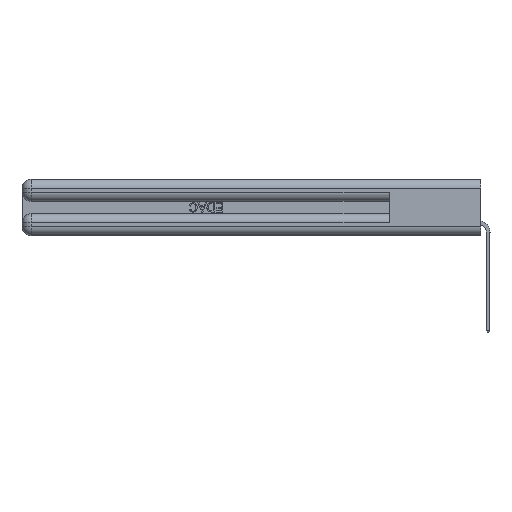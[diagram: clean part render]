
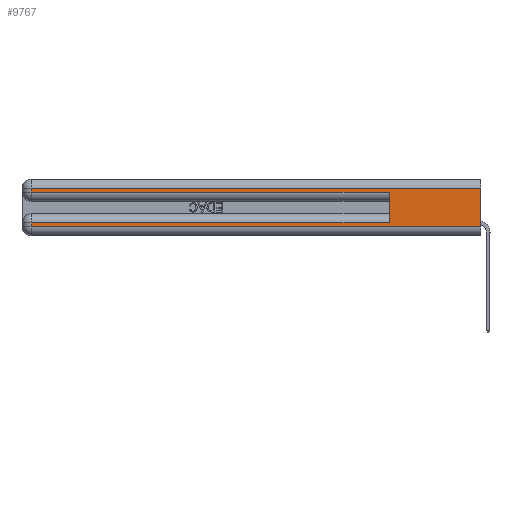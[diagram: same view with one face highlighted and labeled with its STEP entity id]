
A CAD part, left-side view. The second image highlights one B-rep face of the part: STEP entity #9767.
In plain terms, the highlighted planar face has unit normal (-1, 0, 0).
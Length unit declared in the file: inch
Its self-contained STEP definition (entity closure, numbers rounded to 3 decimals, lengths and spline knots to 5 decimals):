
#110 = DIRECTION ( 'NONE',  ( 0., 0., -1. ) ) ;
#471 = ORIENTED_EDGE ( 'NONE', *, *, #6741, .T. ) ;
#808 = DIRECTION ( 'NONE',  ( 0., 1., 0. ) ) ;
#860 = EDGE_LOOP ( 'NONE', ( #19136, #29811, #8137, #3269, #7323, #25403, #471, #20697 ) ) ;
#1047 = CARTESIAN_POINT ( 'NONE',  ( 0., 2.94, 0.285 ) ) ;
#1325 = DIRECTION ( 'NONE',  ( 0., 0., -1. ) ) ;
#2353 = LINE ( 'NONE', #32617, #8210 ) ;
#2904 = CARTESIAN_POINT ( 'NONE',  ( 0., 0., 0.31 ) ) ;
#3269 = ORIENTED_EDGE ( 'NONE', *, *, #11920, .T. ) ;
#3453 = LINE ( 'NONE', #23796, #22189 ) ;
#4743 = CARTESIAN_POINT ( 'NONE',  ( 0., 0., 0.06 ) ) ;
#4805 = VERTEX_POINT ( 'NONE', #20399 ) ;
#5002 = LINE ( 'NONE', #15740, #18308 ) ;
#5163 = DIRECTION ( 'NONE',  ( 0., 1., 0. ) ) ;
#5506 = EDGE_CURVE ( 'NONE', #16180, #24218, #18755, .T. ) ;
#5620 = CARTESIAN_POINT ( 'NONE',  ( 0., 2.94, 0.06 ) ) ;
#6741 = EDGE_CURVE ( 'NONE', #19125, #13672, #11474, .T. ) ;
#7008 = VERTEX_POINT ( 'NONE', #27157 ) ;
#7323 = ORIENTED_EDGE ( 'NONE', *, *, #32659, .F. ) ;
#7396 = VECTOR ( 'NONE', #33219, 39.37008 ) ;
#8137 = ORIENTED_EDGE ( 'NONE', *, *, #32264, .T. ) ;
#8210 = VECTOR ( 'NONE', #23501, 39.37008 ) ;
#8290 = VECTOR ( 'NONE', #28576, 39.37008 ) ;
#9767 = ADVANCED_FACE ( 'NONE', ( #28281 ), #32819, .F. ) ;
#10044 = LINE ( 'NONE', #4743, #26660 ) ;
#10461 = VERTEX_POINT ( 'NONE', #1047 ) ;
#10811 = LINE ( 'NONE', #17543, #8290 ) ;
#11448 = DIRECTION ( 'NONE',  ( 1., 0., 0. ) ) ;
#11470 = EDGE_CURVE ( 'NONE', #16180, #14754, #22353, .T. ) ;
#11474 = LINE ( 'NONE', #33855, #34330 ) ;
#11920 = EDGE_CURVE ( 'NONE', #10461, #4805, #2353, .T. ) ;
#13672 = VERTEX_POINT ( 'NONE', #5620 ) ;
#14106 = CARTESIAN_POINT ( 'NONE',  ( 0., 0., 0.37 ) ) ;
#14754 = VERTEX_POINT ( 'NONE', #23973 ) ;
#14987 = CARTESIAN_POINT ( 'NONE',  ( 0., 0., 0.37 ) ) ;
#15740 = CARTESIAN_POINT ( 'NONE',  ( 0., 2.94, 0.37 ) ) ;
#16180 = VERTEX_POINT ( 'NONE', #29236 ) ;
#17543 = CARTESIAN_POINT ( 'NONE',  ( 0., 0.6, 0.145 ) ) ;
#18182 = AXIS2_PLACEMENT_3D ( 'NONE', #14106, #11448, #1325 ) ;
#18308 = VECTOR ( 'NONE', #110, 39.37008 ) ;
#18755 = LINE ( 'NONE', #2904, #32092 ) ;
#19125 = VERTEX_POINT ( 'NONE', #25546 ) ;
#19136 = ORIENTED_EDGE ( 'NONE', *, *, #11470, .F. ) ;
#19444 = EDGE_CURVE ( 'NONE', #7008, #19125, #3453, .T. ) ;
#20399 = CARTESIAN_POINT ( 'NONE',  ( 0., 0.6, 0.285 ) ) ;
#20570 = DIRECTION ( 'NONE',  ( 0., -1., 0. ) ) ;
#20646 = DIRECTION ( 'NONE',  ( 0., 0., -1. ) ) ;
#20697 = ORIENTED_EDGE ( 'NONE', *, *, #27111, .T. ) ;
#22189 = VECTOR ( 'NONE', #5163, 39.37008 ) ;
#22353 = LINE ( 'NONE', #14987, #7396 ) ;
#22760 = CARTESIAN_POINT ( 'NONE',  ( 0., 2.94, 0.31 ) ) ;
#23501 = DIRECTION ( 'NONE',  ( 0., -1., 0. ) ) ;
#23796 = CARTESIAN_POINT ( 'NONE',  ( 0., 0., 0.085 ) ) ;
#23973 = CARTESIAN_POINT ( 'NONE',  ( 0., 0., 0.06 ) ) ;
#24218 = VERTEX_POINT ( 'NONE', #22760 ) ;
#25403 = ORIENTED_EDGE ( 'NONE', *, *, #19444, .T. ) ;
#25546 = CARTESIAN_POINT ( 'NONE',  ( 0., 2.94, 0.085 ) ) ;
#26660 = VECTOR ( 'NONE', #20570, 39.37008 ) ;
#27111 = EDGE_CURVE ( 'NONE', #13672, #14754, #10044, .T. ) ;
#27157 = CARTESIAN_POINT ( 'NONE',  ( 0., 0.6, 0.085 ) ) ;
#28281 = FACE_OUTER_BOUND ( 'NONE', #860, .T. ) ;
#28576 = DIRECTION ( 'NONE',  ( 0., 0., 1. ) ) ;
#29236 = CARTESIAN_POINT ( 'NONE',  ( 0., 0., 0.31 ) ) ;
#29811 = ORIENTED_EDGE ( 'NONE', *, *, #5506, .T. ) ;
#32092 = VECTOR ( 'NONE', #808, 39.37008 ) ;
#32264 = EDGE_CURVE ( 'NONE', #24218, #10461, #5002, .T. ) ;
#32617 = CARTESIAN_POINT ( 'NONE',  ( 0., 0., 0.285 ) ) ;
#32659 = EDGE_CURVE ( 'NONE', #7008, #4805, #10811, .T. ) ;
#32819 = PLANE ( 'NONE',  #18182 ) ;
#33219 = DIRECTION ( 'NONE',  ( 0., 0., -1. ) ) ;
#33855 = CARTESIAN_POINT ( 'NONE',  ( 0., 2.94, 0.37 ) ) ;
#34330 = VECTOR ( 'NONE', #20646, 39.37008 ) ;
